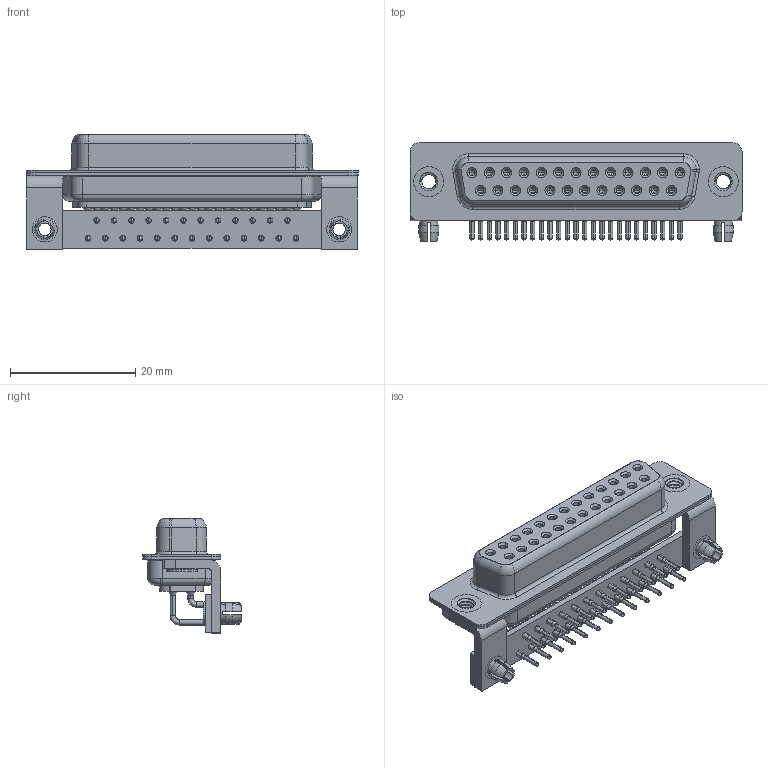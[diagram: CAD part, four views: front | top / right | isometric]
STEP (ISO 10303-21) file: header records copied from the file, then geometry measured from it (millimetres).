
FILE_DESCRIPTION (( 'STEP AP203' ), '1' );
FILE_NAME ('622-M25-660-BT3.STEP', '2018-09-24T22:05:38', ( '' ), ( '' ), 'SwSTEP 2.0', 'SolidWorks 2016', '' );
FILE_SCHEMA (( 'CONFIG_CONTROL_DESIGN' ));
Length unit declared in the file: millimetre
Products named in the file (10): 622M 4-40 Threaded Rivet_Stabilizer; 622M Housing_25 Contacts; 622M Stabilizer Bracket; 622M Shell Front_25 Contacts; 622M Stabilizer Board_25 Contacts; 622M Shell Rear_25 Contacts; 622M Board Lock; 622M Contact Row 1; 622-M25-660-BT3; 622M Contact Row 2
Assembly tree (35 placements, depth 2):
  622-M25-660-BT3
    622M Housing_25 Contacts
    622M Shell Front_25 Contacts
    622M Shell Rear_25 Contacts
    622M Contact Row 1  x13
    622M Contact Row 2  x12
    622M 4-40 Threaded Rivet_Stabilizer  x2
    622M Stabilizer Bracket  x2
    622M Stabilizer Board_25 Contacts
    622M Board Lock  x2
Bounding box: 53.05 x 15.8 x 18.5 mm (x, y, z)
Volume: 4408.1 mm3; surface area: 11042.5 mm2
Topology: 35 solids, 35 shells, 1796 faces, 4586 edges, 2900 vertices
Faces by surface type: cylinder 816, plane 516, cone 295, bspline 106, torus 63
Entity records: 26597 total; most frequent: CARTESIAN_POINT 5709, DIRECTION 4393, ORIENTED_EDGE 3720, EDGE_CURVE 1860, AXIS2_PLACEMENT_3D 1826, VERTEX_POINT 1191, CIRCLE 1022, EDGE_LOOP 991
